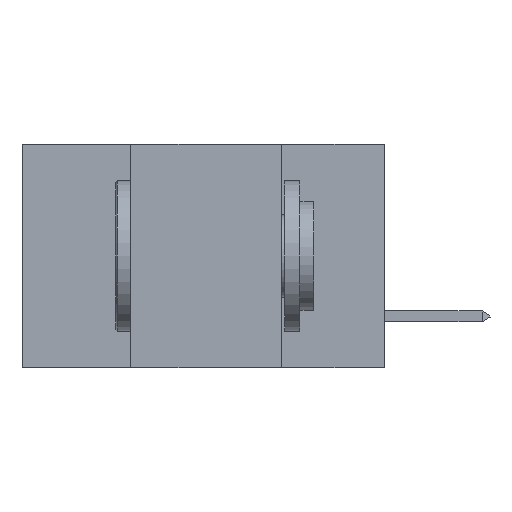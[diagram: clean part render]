
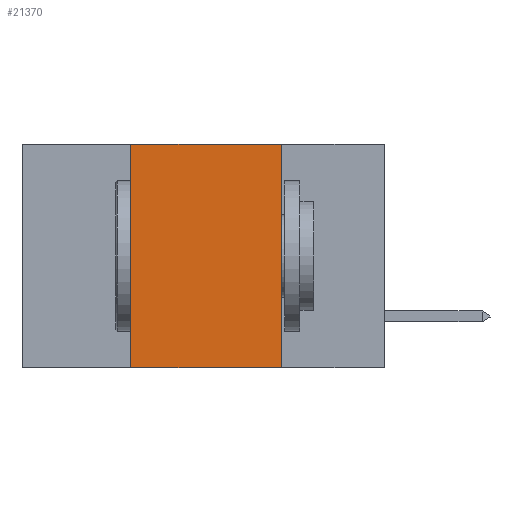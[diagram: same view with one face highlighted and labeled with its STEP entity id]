
A CAD part, left-side view. The second image highlights one B-rep face of the part: STEP entity #21370.
In plain terms, the highlighted planar face has unit normal (-1, 0, 0).
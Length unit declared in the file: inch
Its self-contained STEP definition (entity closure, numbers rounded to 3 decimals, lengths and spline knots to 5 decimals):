
#183 = VERTEX_POINT ( 'NONE', #935 ) ;
#488 = EDGE_LOOP ( 'NONE', ( #4680, #6249, #26689, #19213 ) ) ;
#935 = CARTESIAN_POINT ( 'NONE',  ( 0., 0.42, -0.37 ) ) ;
#1669 = EDGE_CURVE ( 'NONE', #183, #3226, #11669, .T. ) ;
#1811 = VERTEX_POINT ( 'NONE', #7974 ) ;
#3226 = VERTEX_POINT ( 'NONE', #7840 ) ;
#4335 = CARTESIAN_POINT ( 'NONE',  ( 0., 0.42, 0. ) ) ;
#4680 = ORIENTED_EDGE ( 'NONE', *, *, #7164, .F. ) ;
#5117 = CARTESIAN_POINT ( 'NONE',  ( 0., 0.17, 0. ) ) ;
#5295 = LINE ( 'NONE', #4335, #15072 ) ;
#5424 = DIRECTION ( 'NONE',  ( 1., 0., 0. ) ) ;
#5688 = PLANE ( 'NONE',  #6515 ) ;
#6249 = ORIENTED_EDGE ( 'NONE', *, *, #8198, .F. ) ;
#6515 = AXIS2_PLACEMENT_3D ( 'NONE', #17897, #5424, #7331 ) ;
#7164 = EDGE_CURVE ( 'NONE', #15706, #3226, #11562, .T. ) ;
#7331 = DIRECTION ( 'NONE',  ( 0., 0., -1. ) ) ;
#7614 = FACE_OUTER_BOUND ( 'NONE', #488, .T. ) ;
#7840 = CARTESIAN_POINT ( 'NONE',  ( 0., 0.17, -0.37 ) ) ;
#7974 = CARTESIAN_POINT ( 'NONE',  ( 0., 0.42, 0. ) ) ;
#8198 = EDGE_CURVE ( 'NONE', #1811, #15706, #17034, .T. ) ;
#11390 = EDGE_CURVE ( 'NONE', #183, #1811, #5295, .T. ) ;
#11562 = LINE ( 'NONE', #5117, #12550 ) ;
#11669 = LINE ( 'NONE', #14941, #16538 ) ;
#12550 = VECTOR ( 'NONE', #15865, 39.37008 ) ;
#13371 = DIRECTION ( 'NONE',  ( 0., -1., 0. ) ) ;
#14941 = CARTESIAN_POINT ( 'NONE',  ( 0., 0.6, -0.37 ) ) ;
#15072 = VECTOR ( 'NONE', #17001, 39.37008 ) ;
#15706 = VERTEX_POINT ( 'NONE', #19451 ) ;
#15865 = DIRECTION ( 'NONE',  ( 0., 0., -1. ) ) ;
#16538 = VECTOR ( 'NONE', #21844, 39.37008 ) ;
#17001 = DIRECTION ( 'NONE',  ( 0., 0., 1. ) ) ;
#17034 = LINE ( 'NONE', #21546, #17659 ) ;
#17659 = VECTOR ( 'NONE', #13371, 39.37008 ) ;
#17897 = CARTESIAN_POINT ( 'NONE',  ( 0., 0.6, 0. ) ) ;
#19213 = ORIENTED_EDGE ( 'NONE', *, *, #1669, .T. ) ;
#19451 = CARTESIAN_POINT ( 'NONE',  ( 0., 0.17, 0. ) ) ;
#21370 = ADVANCED_FACE ( 'NONE', ( #7614 ), #5688, .F. ) ;
#21546 = CARTESIAN_POINT ( 'NONE',  ( 0., 0.6, 0. ) ) ;
#21844 = DIRECTION ( 'NONE',  ( 0., -1., 0. ) ) ;
#26689 = ORIENTED_EDGE ( 'NONE', *, *, #11390, .F. ) ;
